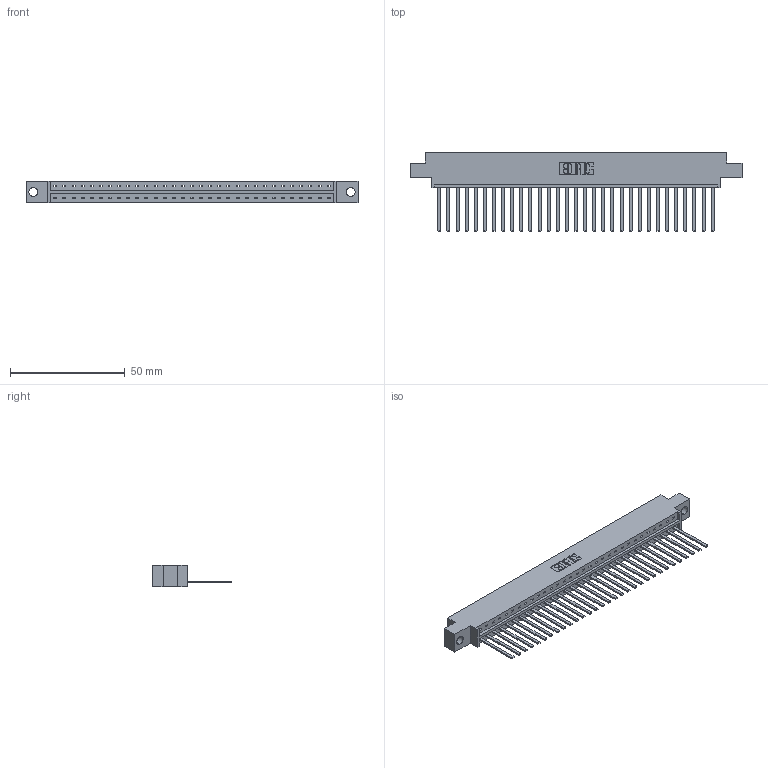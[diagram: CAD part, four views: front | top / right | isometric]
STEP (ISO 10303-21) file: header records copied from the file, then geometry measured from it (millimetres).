
FILE_DESCRIPTION (( 'STEP AP203' ), '1' );
FILE_NAME ('833-031-544-604.STEP', '2020-06-02T15:55:56', ( '' ), ( '' ), 'SwSTEP 2.0', 'SolidWorks 2020', '' );
FILE_SCHEMA (( 'CONFIG_CONTROL_DESIGN' ));
Length unit declared in the file: inch
Products named in the file (3): 345-292-001_345-293-144; 833 Part_Offset - .156 Dia - TH; 833-031-544-604
Assembly tree (32 placements, depth 2):
  833-031-544-604
    833 Part_Offset - .156 Dia - TH
    345-292-001_345-293-144  x31
Bounding box: 144.37 x 34.3 x 9.4 mm (x, y, z)
Volume: 14476.8 mm3; surface area: 16752.5 mm2
Topology: 32 solids, 32 shells, 1730 faces, 5221 edges, 3438 vertices
Faces by surface type: plane 1252, cylinder 478
Entity records: 20325 total; most frequent: CARTESIAN_POINT 3515, ORIENTED_EDGE 3482, DIRECTION 2983, EDGE_CURVE 1741, VECTOR 1617, LINE 1617, VERTEX_POINT 1158, AXIS2_PLACEMENT_3D 683
